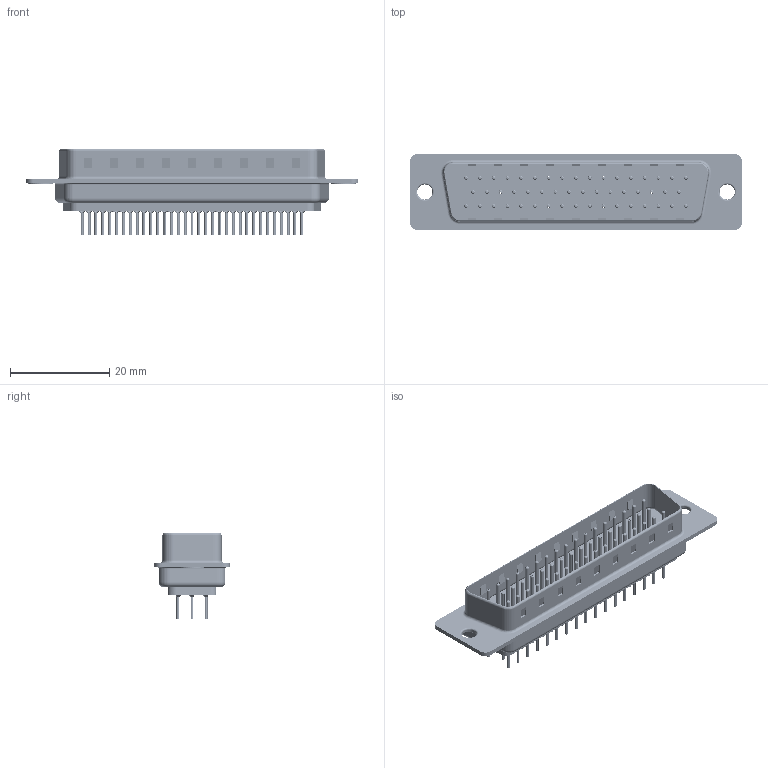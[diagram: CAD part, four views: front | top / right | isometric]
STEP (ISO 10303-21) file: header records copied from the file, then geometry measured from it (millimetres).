
FILE_DESCRIPTION (( 'STEP AP203' ), '1' );
FILE_NAME ('627-050-620-061.STEP', '2020-07-15T15:10:23', ( '' ), ( '' ), 'SwSTEP 2.0', 'SolidWorks 2020', '' );
FILE_SCHEMA (( 'CONFIG_CONTROL_DESIGN' ));
Length unit declared in the file: millimetre
Products named in the file (8): 627 Thru Hole Rivet; 627 Contact Row 3_20L; 627 Contact Row 1_20L; 627 Shell Front_50 Contacts; 627 Housing_50 LP; 627-050-620-061; 627 Contact Row 2_20L; 627 Shell Rear_50 Contacts
Assembly tree (55 placements, depth 2):
  627-050-620-061
    627 Housing_50 LP
    627 Shell Front_50 Contacts
    627 Shell Rear_50 Contacts
    627 Contact Row 1_20L  x17
    627 Contact Row 2_20L  x16
    627 Contact Row 3_20L  x17
    627 Thru Hole Rivet  x2
Bounding box: 67 x 15.3 x 17.3 mm (x, y, z)
Volume: 4346.2 mm3; surface area: 12439.6 mm2
Topology: 55 solids, 55 shells, 5286 faces, 13825 edges, 8560 vertices
Faces by surface type: cylinder 1975, torus 1408, plane 1403, cone 500
Entity records: 34165 total; most frequent: CARTESIAN_POINT 6129, DIRECTION 5884, ORIENTED_EDGE 5080, EDGE_CURVE 2540, AXIS2_PLACEMENT_3D 2361, VERTEX_POINT 1627, EDGE_LOOP 1295, CIRCLE 1267
